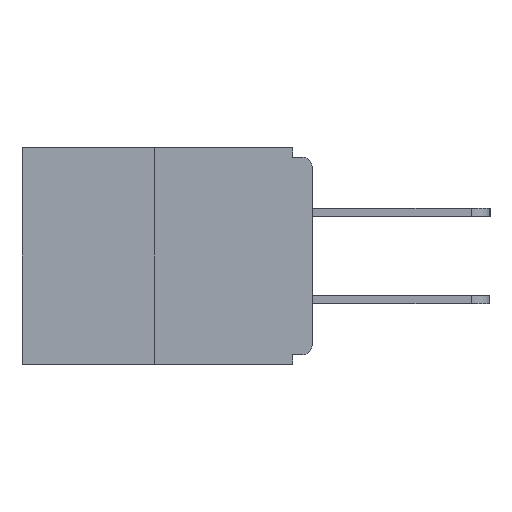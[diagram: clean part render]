
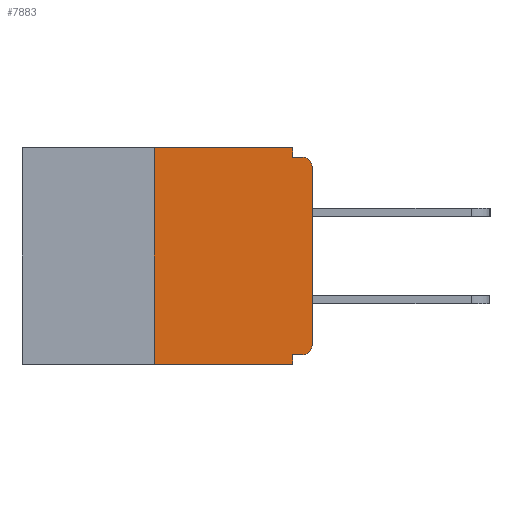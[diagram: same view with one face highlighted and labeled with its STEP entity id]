
A CAD part, left-side view. The second image highlights one B-rep face of the part: STEP entity #7883.
In plain terms, the highlighted planar face has unit normal (-1, 0, 0).
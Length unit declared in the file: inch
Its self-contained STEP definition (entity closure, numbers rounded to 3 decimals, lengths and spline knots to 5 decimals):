
#198 = VECTOR ( 'NONE', #4689, 39.37008 ) ;
#324 = VERTEX_POINT ( 'NONE', #1744 ) ;
#352 = FACE_OUTER_BOUND ( 'NONE', #11369, .T. ) ;
#509 = VERTEX_POINT ( 'NONE', #1154 ) ;
#707 = VECTOR ( 'NONE', #2597, 39.37008 ) ;
#1154 = CARTESIAN_POINT ( 'NONE',  ( 0., 0.031, -0.343 ) ) ;
#1605 = CARTESIAN_POINT ( 'NONE',  ( 0., 0.031, 0. ) ) ;
#1744 = CARTESIAN_POINT ( 'NONE',  ( 0., 0.031, -0.015 ) ) ;
#1828 = CARTESIAN_POINT ( 'NONE',  ( 0., 0.015, -0.313 ) ) ;
#2098 = LINE ( 'NONE', #6558, #707 ) ;
#2597 = DIRECTION ( 'NONE',  ( 0., 0., 1. ) ) ;
#2882 = EDGE_CURVE ( 'NONE', #324, #7634, #16037, .T. ) ;
#2897 = DIRECTION ( 'NONE',  ( 0., 0., -1. ) ) ;
#3307 = CIRCLE ( 'NONE', #9388, 0.015 ) ;
#3402 = DIRECTION ( 'NONE',  ( 1., 0., 0. ) ) ;
#3467 = CARTESIAN_POINT ( 'NONE',  ( 0., 0.46, 0. ) ) ;
#4075 = LINE ( 'NONE', #8116, #198 ) ;
#4150 = VECTOR ( 'NONE', #2897, 39.37008 ) ;
#4385 = VERTEX_POINT ( 'NONE', #4883 ) ;
#4399 = ORIENTED_EDGE ( 'NONE', *, *, #5914, .F. ) ;
#4544 = VERTEX_POINT ( 'NONE', #5013 ) ;
#4578 = CARTESIAN_POINT ( 'NONE',  ( 0., 0.015, -0.015 ) ) ;
#4689 = DIRECTION ( 'NONE',  ( 0., 1., 0. ) ) ;
#4883 = CARTESIAN_POINT ( 'NONE',  ( 0., 0., -0.313 ) ) ;
#5013 = CARTESIAN_POINT ( 'NONE',  ( 0., 0.015, -0.328 ) ) ;
#5608 = ORIENTED_EDGE ( 'NONE', *, *, #2882, .F. ) ;
#5716 = DIRECTION ( 'NONE',  ( 0., 0., -1. ) ) ;
#5811 = ORIENTED_EDGE ( 'NONE', *, *, #9546, .T. ) ;
#5914 = EDGE_CURVE ( 'NONE', #4544, #10208, #4075, .T. ) ;
#6080 = ORIENTED_EDGE ( 'NONE', *, *, #15831, .F. ) ;
#6156 = DIRECTION ( 'NONE',  ( 0., 0., -1. ) ) ;
#6258 = ORIENTED_EDGE ( 'NONE', *, *, #15650, .F. ) ;
#6382 = DIRECTION ( 'NONE',  ( -1., 0., 0. ) ) ;
#6514 = VERTEX_POINT ( 'NONE', #11734 ) ;
#6558 = CARTESIAN_POINT ( 'NONE',  ( 0., 0., 0. ) ) ;
#6796 = DIRECTION ( 'NONE',  ( -1., 0., 0. ) ) ;
#6857 = DIRECTION ( 'NONE',  ( 0., -1., 0. ) ) ;
#7246 = PLANE ( 'NONE',  #12561 ) ;
#7608 = LINE ( 'NONE', #1605, #4150 ) ;
#7634 = VERTEX_POINT ( 'NONE', #4578 ) ;
#7807 = LINE ( 'NONE', #15050, #11079 ) ;
#7860 = EDGE_CURVE ( 'NONE', #6514, #509, #15867, .T. ) ;
#7883 = ADVANCED_FACE ( 'NONE', ( #352 ), #7246, .F. ) ;
#8000 = CIRCLE ( 'NONE', #12725, 0.015 ) ;
#8116 = CARTESIAN_POINT ( 'NONE',  ( 0., 0., -0.328 ) ) ;
#8221 = DIRECTION ( 'NONE',  ( 0., 0., -1. ) ) ;
#8559 = ORIENTED_EDGE ( 'NONE', *, *, #7860, .T. ) ;
#9076 = VECTOR ( 'NONE', #6857, 39.37008 ) ;
#9091 = EDGE_CURVE ( 'NONE', #6514, #12872, #15205, .T. ) ;
#9236 = ORIENTED_EDGE ( 'NONE', *, *, #10921, .F. ) ;
#9249 = CARTESIAN_POINT ( 'NONE',  ( 0., 0., -0.03 ) ) ;
#9329 = ORIENTED_EDGE ( 'NONE', *, *, #9091, .F. ) ;
#9388 = AXIS2_PLACEMENT_3D ( 'NONE', #10190, #6382, #6156 ) ;
#9546 = EDGE_CURVE ( 'NONE', #4385, #11686, #2098, .T. ) ;
#9622 = CARTESIAN_POINT ( 'NONE',  ( 0., 0.46, -0.343 ) ) ;
#9901 = CARTESIAN_POINT ( 'NONE',  ( 0., 0.031, -0.328 ) ) ;
#10093 = VECTOR ( 'NONE', #14737, 39.37008 ) ;
#10129 = EDGE_CURVE ( 'NONE', #4544, #4385, #8000, .T. ) ;
#10190 = CARTESIAN_POINT ( 'NONE',  ( 0., 0.015, -0.03 ) ) ;
#10208 = VERTEX_POINT ( 'NONE', #9901 ) ;
#10477 = CARTESIAN_POINT ( 'NONE',  ( 0., 0.031, 0. ) ) ;
#10828 = EDGE_CURVE ( 'NONE', #11686, #7634, #3307, .T. ) ;
#10921 = EDGE_CURVE ( 'NONE', #10208, #509, #16383, .T. ) ;
#11006 = ORIENTED_EDGE ( 'NONE', *, *, #10828, .T. ) ;
#11079 = VECTOR ( 'NONE', #15153, 39.37008 ) ;
#11369 = EDGE_LOOP ( 'NONE', ( #6080, #9329, #8559, #9236, #4399, #15445, #5811, #11006, #5608, #6258 ) ) ;
#11686 = VERTEX_POINT ( 'NONE', #9249 ) ;
#11734 = CARTESIAN_POINT ( 'NONE',  ( 0., 0.25, -0.343 ) ) ;
#12561 = AXIS2_PLACEMENT_3D ( 'NONE', #3467, #3402, #12658 ) ;
#12658 = DIRECTION ( 'NONE',  ( 0., 0., -1. ) ) ;
#12725 = AXIS2_PLACEMENT_3D ( 'NONE', #1828, #6796, #5716 ) ;
#12872 = VERTEX_POINT ( 'NONE', #15839 ) ;
#12874 = VECTOR ( 'NONE', #8221, 39.37008 ) ;
#13322 = CARTESIAN_POINT ( 'NONE',  ( 0., 0.25, 0. ) ) ;
#13437 = DIRECTION ( 'NONE',  ( 0., -1., 0. ) ) ;
#14729 = CARTESIAN_POINT ( 'NONE',  ( 0., 0., -0.015 ) ) ;
#14737 = DIRECTION ( 'NONE',  ( 0., 0., 1. ) ) ;
#14985 = VERTEX_POINT ( 'NONE', #10477 ) ;
#15050 = CARTESIAN_POINT ( 'NONE',  ( 0., 0.46, 0. ) ) ;
#15153 = DIRECTION ( 'NONE',  ( 0., -1., 0. ) ) ;
#15205 = LINE ( 'NONE', #13322, #10093 ) ;
#15445 = ORIENTED_EDGE ( 'NONE', *, *, #10129, .T. ) ;
#15597 = CARTESIAN_POINT ( 'NONE',  ( 0., 0.031, -0.343 ) ) ;
#15650 = EDGE_CURVE ( 'NONE', #14985, #324, #7608, .T. ) ;
#15831 = EDGE_CURVE ( 'NONE', #12872, #14985, #7807, .T. ) ;
#15839 = CARTESIAN_POINT ( 'NONE',  ( 0., 0.25, 0. ) ) ;
#15867 = LINE ( 'NONE', #9622, #16685 ) ;
#16037 = LINE ( 'NONE', #14729, #9076 ) ;
#16383 = LINE ( 'NONE', #15597, #12874 ) ;
#16685 = VECTOR ( 'NONE', #13437, 39.37008 ) ;
